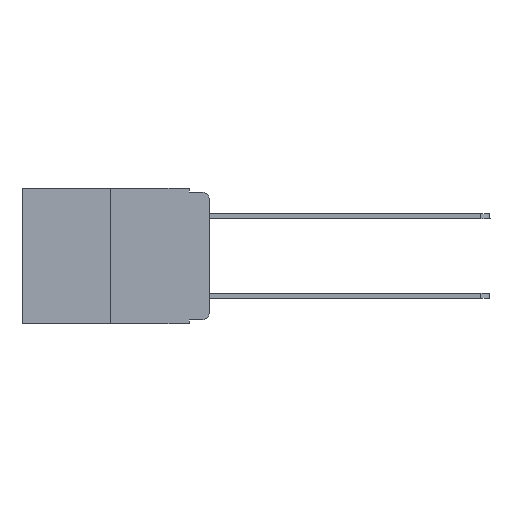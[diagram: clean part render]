
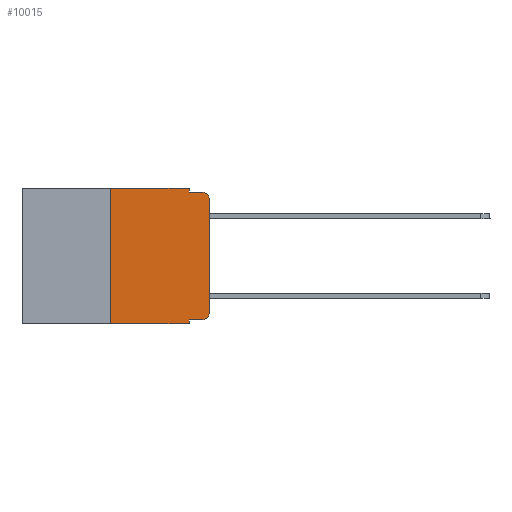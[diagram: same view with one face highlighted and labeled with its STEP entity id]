
A CAD part, left-side view. The second image highlights one B-rep face of the part: STEP entity #10015.
In plain terms, the highlighted planar face has unit normal (-1, 0, 0).
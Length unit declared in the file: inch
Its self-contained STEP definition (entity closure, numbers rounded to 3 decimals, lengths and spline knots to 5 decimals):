
#275 = ORIENTED_EDGE ( 'NONE', *, *, #3640, .F. ) ;
#451 = VERTEX_POINT ( 'NONE', #10224 ) ;
#593 = EDGE_CURVE ( 'NONE', #5125, #7509, #7524, .T. ) ;
#616 = VERTEX_POINT ( 'NONE', #14853 ) ;
#845 = VERTEX_POINT ( 'NONE', #12829 ) ;
#1107 = VECTOR ( 'NONE', #5655, 39.37008 ) ;
#1423 = VECTOR ( 'NONE', #16966, 39.37008 ) ;
#1619 = VERTEX_POINT ( 'NONE', #4200 ) ;
#2086 = EDGE_CURVE ( 'NONE', #451, #845, #4845, .T. ) ;
#2130 = DIRECTION ( 'NONE',  ( -1., 0., 0. ) ) ;
#2304 = DIRECTION ( 'NONE',  ( 0., 0., -1. ) ) ;
#2576 = VECTOR ( 'NONE', #9968, 39.37008 ) ;
#2775 = PLANE ( 'NONE',  #5782 ) ;
#2873 = CARTESIAN_POINT ( 'NONE',  ( 0., 0.051, 0. ) ) ;
#3571 = CIRCLE ( 'NONE', #17517, 0.02 ) ;
#3640 = EDGE_CURVE ( 'NONE', #616, #6014, #3667, .T. ) ;
#3667 = LINE ( 'NONE', #8544, #2576 ) ;
#3725 = CARTESIAN_POINT ( 'NONE',  ( 0., 0.02, -0.313 ) ) ;
#3984 = DIRECTION ( 'NONE',  ( 1., 0., 0. ) ) ;
#4055 = VERTEX_POINT ( 'NONE', #14803 ) ;
#4200 = CARTESIAN_POINT ( 'NONE',  ( 0., 0.051, -0.343 ) ) ;
#4207 = EDGE_CURVE ( 'NONE', #7509, #451, #3571, .T. ) ;
#4271 = LINE ( 'NONE', #4626, #5793 ) ;
#4626 = CARTESIAN_POINT ( 'NONE',  ( 0., 0.473, 0. ) ) ;
#4845 = LINE ( 'NONE', #6991, #1107 ) ;
#4885 = CARTESIAN_POINT ( 'NONE',  ( 0., 0.02, -0.03 ) ) ;
#4990 = DIRECTION ( 'NONE',  ( 0., -1., 0. ) ) ;
#5125 = VERTEX_POINT ( 'NONE', #16909 ) ;
#5245 = FACE_OUTER_BOUND ( 'NONE', #17432, .T. ) ;
#5308 = DIRECTION ( 'NONE',  ( 0., -1., 0. ) ) ;
#5403 = DIRECTION ( 'NONE',  ( 0., 0., -1. ) ) ;
#5456 = VECTOR ( 'NONE', #10164, 39.37008 ) ;
#5642 = ORIENTED_EDGE ( 'NONE', *, *, #2086, .T. ) ;
#5655 = DIRECTION ( 'NONE',  ( 0., 0., 1. ) ) ;
#5782 = AXIS2_PLACEMENT_3D ( 'NONE', #12410, #3984, #5403 ) ;
#5793 = VECTOR ( 'NONE', #4990, 39.37008 ) ;
#6014 = VERTEX_POINT ( 'NONE', #12528 ) ;
#6103 = ORIENTED_EDGE ( 'NONE', *, *, #593, .T. ) ;
#6991 = CARTESIAN_POINT ( 'NONE',  ( 0., 0., 0. ) ) ;
#7304 = ORIENTED_EDGE ( 'NONE', *, *, #14676, .F. ) ;
#7463 = AXIS2_PLACEMENT_3D ( 'NONE', #4885, #2130, #2304 ) ;
#7496 = EDGE_CURVE ( 'NONE', #13645, #1619, #12612, .T. ) ;
#7509 = VERTEX_POINT ( 'NONE', #8520 ) ;
#7524 = LINE ( 'NONE', #13059, #16976 ) ;
#7535 = LINE ( 'NONE', #2873, #13936 ) ;
#7591 = EDGE_CURVE ( 'NONE', #5125, #1619, #7535, .T. ) ;
#8196 = LINE ( 'NONE', #9677, #1423 ) ;
#8306 = LINE ( 'NONE', #17170, #5456 ) ;
#8520 = CARTESIAN_POINT ( 'NONE',  ( 0., 0.02, -0.333 ) ) ;
#8544 = CARTESIAN_POINT ( 'NONE',  ( 0., 0.051, -0.01 ) ) ;
#8633 = ORIENTED_EDGE ( 'NONE', *, *, #14879, .F. ) ;
#9253 = VERTEX_POINT ( 'NONE', #13504 ) ;
#9277 = DIRECTION ( 'NONE',  ( 0., -1., 0. ) ) ;
#9677 = CARTESIAN_POINT ( 'NONE',  ( 0., 0.25, 0. ) ) ;
#9968 = DIRECTION ( 'NONE',  ( 0., -1., 0. ) ) ;
#10015 = ADVANCED_FACE ( 'NONE', ( #5245 ), #2775, .F. ) ;
#10164 = DIRECTION ( 'NONE',  ( 0., 0., -1. ) ) ;
#10224 = CARTESIAN_POINT ( 'NONE',  ( 0., 0., -0.313 ) ) ;
#10573 = ORIENTED_EDGE ( 'NONE', *, *, #11421, .F. ) ;
#10986 = EDGE_CURVE ( 'NONE', #845, #6014, #14714, .T. ) ;
#11421 = EDGE_CURVE ( 'NONE', #4055, #616, #8306, .T. ) ;
#12149 = VECTOR ( 'NONE', #5308, 39.37008 ) ;
#12410 = CARTESIAN_POINT ( 'NONE',  ( 0., 0.473, 0. ) ) ;
#12528 = CARTESIAN_POINT ( 'NONE',  ( 0., 0.02, -0.01 ) ) ;
#12612 = LINE ( 'NONE', #17908, #12149 ) ;
#12729 = DIRECTION ( 'NONE',  ( 0., 0., -1. ) ) ;
#12829 = CARTESIAN_POINT ( 'NONE',  ( 0., 0., -0.03 ) ) ;
#13059 = CARTESIAN_POINT ( 'NONE',  ( 0., 0.051, -0.333 ) ) ;
#13504 = CARTESIAN_POINT ( 'NONE',  ( 0., 0.25, 0. ) ) ;
#13597 = DIRECTION ( 'NONE',  ( -1., 0., 0. ) ) ;
#13625 = ORIENTED_EDGE ( 'NONE', *, *, #10986, .T. ) ;
#13645 = VERTEX_POINT ( 'NONE', #17201 ) ;
#13757 = DIRECTION ( 'NONE',  ( 0., 0., -1. ) ) ;
#13936 = VECTOR ( 'NONE', #12729, 39.37008 ) ;
#14050 = ORIENTED_EDGE ( 'NONE', *, *, #7496, .T. ) ;
#14669 = ORIENTED_EDGE ( 'NONE', *, *, #7591, .F. ) ;
#14676 = EDGE_CURVE ( 'NONE', #13645, #9253, #8196, .T. ) ;
#14714 = CIRCLE ( 'NONE', #7463, 0.02 ) ;
#14803 = CARTESIAN_POINT ( 'NONE',  ( 0., 0.051, 0. ) ) ;
#14853 = CARTESIAN_POINT ( 'NONE',  ( 0., 0.051, -0.01 ) ) ;
#14879 = EDGE_CURVE ( 'NONE', #9253, #4055, #4271, .T. ) ;
#16909 = CARTESIAN_POINT ( 'NONE',  ( 0., 0.051, -0.333 ) ) ;
#16966 = DIRECTION ( 'NONE',  ( 0., 0., 1. ) ) ;
#16976 = VECTOR ( 'NONE', #9277, 39.37008 ) ;
#17170 = CARTESIAN_POINT ( 'NONE',  ( 0., 0.051, 0. ) ) ;
#17201 = CARTESIAN_POINT ( 'NONE',  ( 0., 0.25, -0.343 ) ) ;
#17432 = EDGE_LOOP ( 'NONE', ( #5642, #13625, #275, #10573, #8633, #7304, #14050, #14669, #6103, #18181 ) ) ;
#17517 = AXIS2_PLACEMENT_3D ( 'NONE', #3725, #13597, #13757 ) ;
#17908 = CARTESIAN_POINT ( 'NONE',  ( 0., 0.473, -0.343 ) ) ;
#18181 = ORIENTED_EDGE ( 'NONE', *, *, #4207, .T. ) ;
